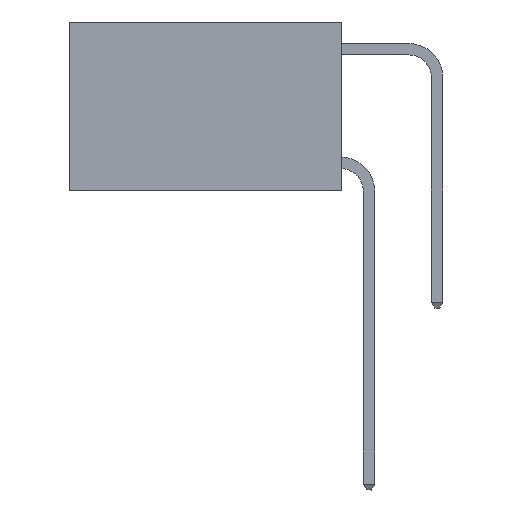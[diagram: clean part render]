
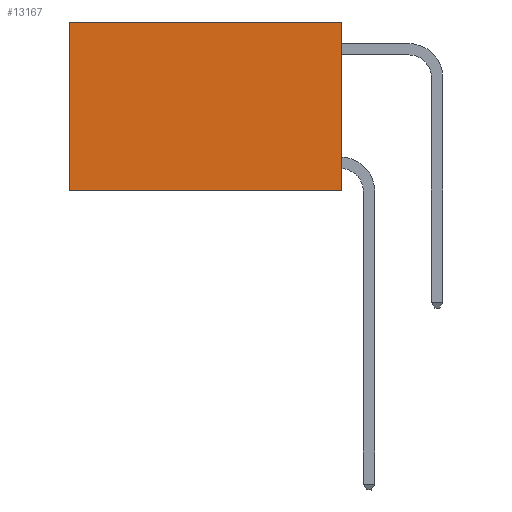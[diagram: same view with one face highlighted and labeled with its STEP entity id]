
A CAD part, left-side view. The second image highlights one B-rep face of the part: STEP entity #13167.
In plain terms, the highlighted planar face has unit normal (-1, 0, 0).
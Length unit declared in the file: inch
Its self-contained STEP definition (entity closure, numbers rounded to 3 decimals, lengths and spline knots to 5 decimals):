
#1258 = LINE ( 'NONE', #4958, #9480 ) ;
#1508 = CARTESIAN_POINT ( 'NONE',  ( 0.2625, 0., 0. ) ) ;
#2164 = VECTOR ( 'NONE', #5741, 39.37008 ) ;
#3553 = EDGE_CURVE ( 'NONE', #11939, #20445, #19969, .T. ) ;
#4336 = VERTEX_POINT ( 'NONE', #22254 ) ;
#4958 = CARTESIAN_POINT ( 'NONE',  ( 0.2625, 0.6, 0. ) ) ;
#5467 = ORIENTED_EDGE ( 'NONE', *, *, #3553, .F. ) ;
#5741 = DIRECTION ( 'NONE',  ( 0., 0., -1. ) ) ;
#7063 = PLANE ( 'NONE',  #7998 ) ;
#7538 = ORIENTED_EDGE ( 'NONE', *, *, #17086, .T. ) ;
#7998 = AXIS2_PLACEMENT_3D ( 'NONE', #13489, #15369, #12289 ) ;
#8473 = CARTESIAN_POINT ( 'NONE',  ( 0.2625, 0., 0. ) ) ;
#9480 = VECTOR ( 'NONE', #12060, 39.37008 ) ;
#10948 = EDGE_LOOP ( 'NONE', ( #19267, #12005, #5467, #7538 ) ) ;
#11939 = VERTEX_POINT ( 'NONE', #20402 ) ;
#11953 = FACE_OUTER_BOUND ( 'NONE', #10948, .T. ) ;
#12005 = ORIENTED_EDGE ( 'NONE', *, *, #19798, .F. ) ;
#12060 = DIRECTION ( 'NONE',  ( 0., 0., -1. ) ) ;
#12289 = DIRECTION ( 'NONE',  ( 0., 0., -1. ) ) ;
#12308 = VECTOR ( 'NONE', #22471, 39.37008 ) ;
#12580 = VECTOR ( 'NONE', #20001, 39.37008 ) ;
#13167 = ADVANCED_FACE ( 'NONE', ( #11953 ), #7063, .F. ) ;
#13489 = CARTESIAN_POINT ( 'NONE',  ( 0.2625, 0., 0. ) ) ;
#14511 = LINE ( 'NONE', #21897, #12580 ) ;
#15369 = DIRECTION ( 'NONE',  ( 1., 0., 0. ) ) ;
#15881 = LINE ( 'NONE', #8473, #12308 ) ;
#17086 = EDGE_CURVE ( 'NONE', #11939, #4336, #15881, .T. ) ;
#18017 = VERTEX_POINT ( 'NONE', #21827 ) ;
#18795 = EDGE_CURVE ( 'NONE', #4336, #18017, #1258, .T. ) ;
#19267 = ORIENTED_EDGE ( 'NONE', *, *, #18795, .T. ) ;
#19798 = EDGE_CURVE ( 'NONE', #20445, #18017, #14511, .T. ) ;
#19969 = LINE ( 'NONE', #1508, #2164 ) ;
#20001 = DIRECTION ( 'NONE',  ( 0., 1., 0. ) ) ;
#20402 = CARTESIAN_POINT ( 'NONE',  ( 0.2625, 0., 0. ) ) ;
#20445 = VERTEX_POINT ( 'NONE', #22669 ) ;
#21827 = CARTESIAN_POINT ( 'NONE',  ( 0.2625, 0.6, -0.37 ) ) ;
#21897 = CARTESIAN_POINT ( 'NONE',  ( 0.2625, 0., -0.37 ) ) ;
#22254 = CARTESIAN_POINT ( 'NONE',  ( 0.2625, 0.6, 0. ) ) ;
#22471 = DIRECTION ( 'NONE',  ( 0., 1., 0. ) ) ;
#22669 = CARTESIAN_POINT ( 'NONE',  ( 0.2625, 0., -0.37 ) ) ;
